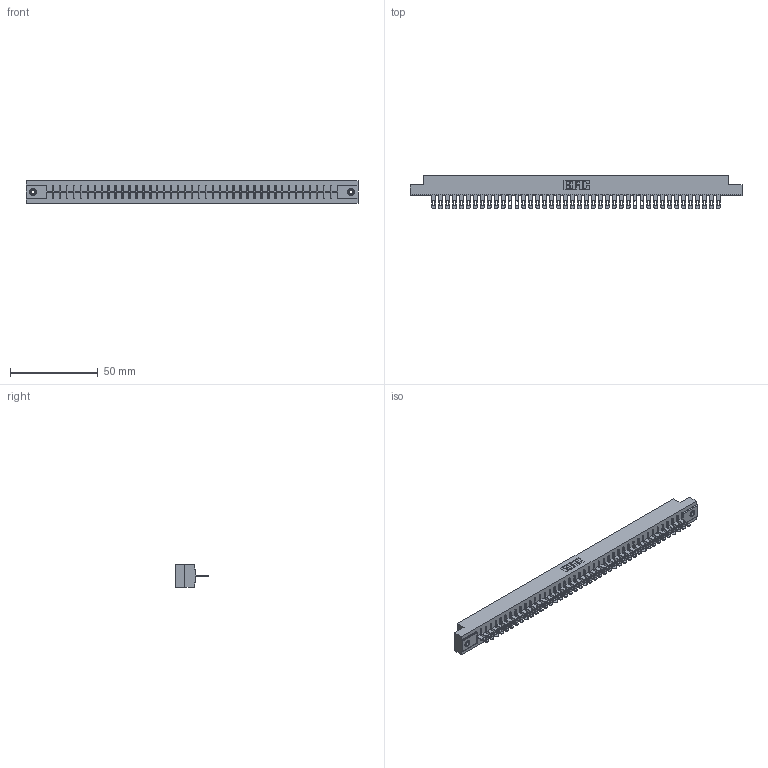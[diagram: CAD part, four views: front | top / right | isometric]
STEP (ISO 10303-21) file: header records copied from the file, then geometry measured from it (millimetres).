
FILE_DESCRIPTION (( 'STEP AP203' ), '1' );
FILE_NAME ('356-042-500-108.STEP', '2018-08-01T22:53:00', ( '' ), ( '' ), 'SwSTEP 2.0', 'SolidWorks 2016', '' );
FILE_SCHEMA (( 'CONFIG_CONTROL_DESIGN' ));
Length unit declared in the file: inch
Products named in the file (4): 306 Part_.156 Dia; 306-290-001_100; 345-250-001_345-250-003-102; 356-042-500-108
Assembly tree (45 placements, depth 2):
  356-042-500-108
    306 Part_.156 Dia
    306-290-001_100  x42
    345-250-001_345-250-003-102  x2
Bounding box: 189.43 x 18.87 x 12.7 mm (x, y, z)
Volume: 21078.1 mm3; surface area: 22400.1 mm2
Topology: 45 solids, 45 shells, 3368 faces, 9482 edges, 6088 vertices
Faces by surface type: plane 2200, cylinder 984, sphere 168, cone 12, torus 4
Entity records: 40516 total; most frequent: CARTESIAN_POINT 6784, ORIENTED_EDGE 6720, DIRECTION 6698, EDGE_CURVE 3360, LINE 2626, VECTOR 2626, VERTEX_POINT 2122, AXIS2_PLACEMENT_3D 2036
